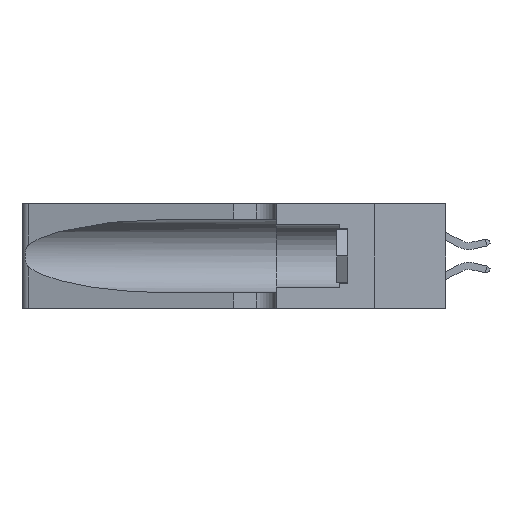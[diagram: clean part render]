
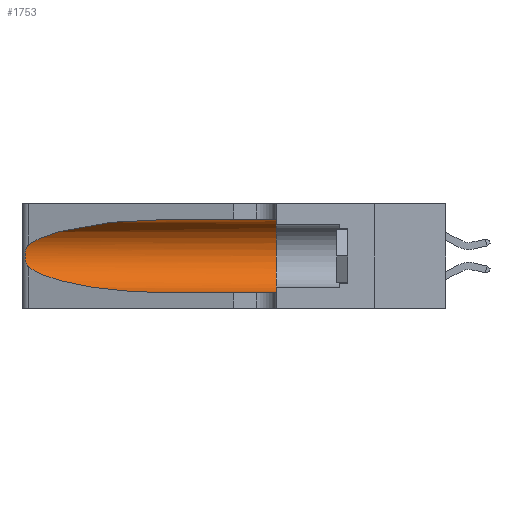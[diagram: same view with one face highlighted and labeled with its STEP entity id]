
A CAD part, left-side view. The second image highlights one B-rep face of the part: STEP entity #1753.
In plain terms, the highlighted cylindrical face has radius 3.308 mm (diameter 6.617 mm), a partial arc.
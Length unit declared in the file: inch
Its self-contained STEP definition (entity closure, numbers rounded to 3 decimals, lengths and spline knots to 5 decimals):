
#166 = CARTESIAN_POINT ( 'NONE',  ( 0.1305, 1.61858, 0.31525 ) ) ;
#1606 = CARTESIAN_POINT ( 'NONE',  ( 0.25787, 1.23484, 0.2124 ) ) ;
#1734 = DIRECTION ( 'NONE',  ( 0., -1., 0. ) ) ;
#1753 = ADVANCED_FACE ( 'NONE', ( #5820 ), #12730, .F. ) ;
#1966 = VERTEX_POINT ( 'NONE', #6187 ) ;
#2011 = CARTESIAN_POINT ( 'NONE',  ( 0.25789, 1.23486, 0.15765 ) ) ;
#2550 = CARTESIAN_POINT ( 'NONE',  ( 0.2373, 1.15595, 0.28018 ) ) ;
#2627 = CARTESIAN_POINT ( 'NONE',  ( 0.25487, 1.22718, 0.22369 ) ) ;
#2708 = DIRECTION ( 'NONE',  ( 0., -1., 0. ) ) ;
#2773 = CARTESIAN_POINT ( 'NONE',  ( 0.18966, 0.96281, 0.31525 ) ) ;
#2777 = CARTESIAN_POINT ( 'NONE',  ( 0.1305, 0.35, 0.31525 ) ) ;
#2837 = CARTESIAN_POINT ( 'NONE',  ( 0.1305, 1.61858, 0.05475 ) ) ;
#3177 = CARTESIAN_POINT ( 'NONE',  ( 0.25487, 1.22718, 0.22369 ) ) ;
#3233 = EDGE_CURVE ( 'NONE', #6096, #1966, #14390, .T. ) ;
#3530 = CARTESIAN_POINT ( 'NONE',  ( 0.26075, 1.23896, 0.178 ) ) ;
#3656 = EDGE_CURVE ( 'NONE', #18512, #18180, #18184, .T. ) ;
#4470 = EDGE_CURVE ( 'NONE', #15712, #6096, #6181, .T. ) ;
#4578 = CARTESIAN_POINT ( 'NONE',  ( 0.1305, 0.35, 0.185 ) ) ;
#5177 = CARTESIAN_POINT ( 'NONE',  ( 0.25555, 1.22993, 0.14849 ) ) ;
#5300 = CARTESIAN_POINT ( 'NONE',  ( 0.18966, 0.96281, 0.05475 ) ) ;
#5494 = EDGE_CURVE ( 'NONE', #18180, #12734, #14915, .T. ) ;
#5590 = ORIENTED_EDGE ( 'NONE', *, *, #3656, .T. ) ;
#5703 = VECTOR ( 'NONE', #1734, 39.37008 ) ;
#5820 = FACE_OUTER_BOUND ( 'NONE', #9398, .T. ) ;
#6096 = VERTEX_POINT ( 'NONE', #2777 ) ;
#6158 = DIRECTION ( 'NONE',  ( 0., 1., 0. ) ) ;
#6181 = LINE ( 'NONE', #166, #5703 ) ;
#6187 = CARTESIAN_POINT ( 'NONE',  ( 0.1305, 0.35, 0.05475 ) ) ;
#6340 = CARTESIAN_POINT ( 'NONE',  ( 0.25854, 1.2359, 0.20912 ) ) ;
#6925 = ORIENTED_EDGE ( 'NONE', *, *, #14265, .T. ) ;
#7083 = AXIS2_PLACEMENT_3D ( 'NONE', #10481, #2708, #7598 ) ;
#7598 = DIRECTION ( 'NONE',  ( 0., 0., -1. ) ) ;
#7863 = ORIENTED_EDGE ( 'NONE', *, *, #3233, .F. ) ;
#9297 = ORIENTED_EDGE ( 'NONE', *, *, #18675, .T. ) ;
#9398 = EDGE_LOOP ( 'NONE', ( #9297, #5590, #18698, #6925, #7863, #17786 ) ) ;
#9500 = CARTESIAN_POINT ( 'NONE',  ( 0.25487, 1.22718, 0.22369 ) ) ;
#9824 = CARTESIAN_POINT ( 'NONE',  ( 0.25639, 1.23186, 0.15144 ) ) ;
#9967 = CARTESIAN_POINT ( 'NONE',  ( 0.26075, 1.23896, 0.19203 ) ) ;
#10028 = CARTESIAN_POINT ( 'NONE',  ( 0.1305, 0.72297, 0.05475 ) ) ;
#10481 = CARTESIAN_POINT ( 'NONE',  ( 0.1305, 1.61858, 0.185 ) ) ;
#10808 = AXIS2_PLACEMENT_3D ( 'NONE', #4578, #6158, #11339 ) ;
#11093 = CARTESIAN_POINT ( 'NONE',  ( 0.25639, 1.23184, 0.21858 ) ) ;
#11285 = LINE ( 'NONE', #2837, #14980 ) ;
#11339 = DIRECTION ( 'NONE',  ( 0., 0., 1. ) ) ;
#12657 = CARTESIAN_POINT ( 'NONE',  ( 0.25487, 1.22718, 0.14631 ) ) ;
#12730 = CYLINDRICAL_SURFACE ( 'NONE', #7083, 0.13025 ) ;
#12734 = VERTEX_POINT ( 'NONE', #14935 ) ;
#12975 = CARTESIAN_POINT ( 'NONE',  ( 0.26018, 1.23835, 0.19895 ) ) ;
#13032 =( BOUNDED_CURVE ( )  B_SPLINE_CURVE ( 3, ( #19920, #2773, #2550, #2627 ),
 .UNSPECIFIED., .F., .T. ) 
 B_SPLINE_CURVE_WITH_KNOTS ( ( 4, 4 ),
 ( 1.5708, 2.84003 ),
 .UNSPECIFIED. ) 
 CURVE ( )  GEOMETRIC_REPRESENTATION_ITEM ( )  RATIONAL_B_SPLINE_CURVE ( ( 1., 0.87, 0.87, 1. ) ) 
 REPRESENTATION_ITEM ( '' )  );
#13180 = CARTESIAN_POINT ( 'NONE',  ( 0.25856, 1.23593, 0.16098 ) ) ;
#14265 = EDGE_CURVE ( 'NONE', #12734, #1966, #11285, .T. ) ;
#14390 = CIRCLE ( 'NONE', #10808, 0.13025 ) ;
#14883 = CARTESIAN_POINT ( 'NONE',  ( 0.25487, 1.22718, 0.14631 ) ) ;
#14915 =( BOUNDED_CURVE ( )  B_SPLINE_CURVE ( 3, ( #12657, #18530, #5300, #10028 ),
 .UNSPECIFIED., .F., .F. ) 
 B_SPLINE_CURVE_WITH_KNOTS ( ( 4, 4 ),
 ( 3.44316, 4.71239 ),
 .UNSPECIFIED. ) 
 CURVE ( )  GEOMETRIC_REPRESENTATION_ITEM ( )  RATIONAL_B_SPLINE_CURVE ( ( 1., 0.87, 0.87, 1. ) ) 
 REPRESENTATION_ITEM ( '' )  );
#14935 = CARTESIAN_POINT ( 'NONE',  ( 0.1305, 0.72297, 0.05475 ) ) ;
#14980 = VECTOR ( 'NONE', #17223, 39.37008 ) ;
#15712 = VERTEX_POINT ( 'NONE', #16688 ) ;
#16058 = CARTESIAN_POINT ( 'NONE',  ( 0.25487, 1.22718, 0.14631 ) ) ;
#16125 = CARTESIAN_POINT ( 'NONE',  ( 0.26017, 1.23833, 0.17102 ) ) ;
#16688 = CARTESIAN_POINT ( 'NONE',  ( 0.1305, 0.72297, 0.31525 ) ) ;
#17223 = DIRECTION ( 'NONE',  ( 0., -1., 0. ) ) ;
#17506 = CARTESIAN_POINT ( 'NONE',  ( 0.25555, 1.22994, 0.2215 ) ) ;
#17786 = ORIENTED_EDGE ( 'NONE', *, *, #4470, .F. ) ;
#18180 = VERTEX_POINT ( 'NONE', #14883 ) ;
#18184 = B_SPLINE_CURVE_WITH_KNOTS ( 'NONE', 3,
 ( #9500, #17506, #11093, #1606, #6340, #12975, #9967, #3530, #16125, #13180, #2011, #9824, #5177, #16058 ),
 .UNSPECIFIED., .F., .F.,
 ( 4, 2, 2, 2, 2, 2, 4 ),
 ( 0., 0.00027, 0.00053, 0.00107, 0.0016, 0.00187, 0.00214 ),
 .UNSPECIFIED. ) ;
#18512 = VERTEX_POINT ( 'NONE', #3177 ) ;
#18530 = CARTESIAN_POINT ( 'NONE',  ( 0.2373, 1.15595, 0.08982 ) ) ;
#18675 = EDGE_CURVE ( 'NONE', #15712, #18512, #13032, .T. ) ;
#18698 = ORIENTED_EDGE ( 'NONE', *, *, #5494, .T. ) ;
#19920 = CARTESIAN_POINT ( 'NONE',  ( 0.1305, 0.72297, 0.31525 ) ) ;
